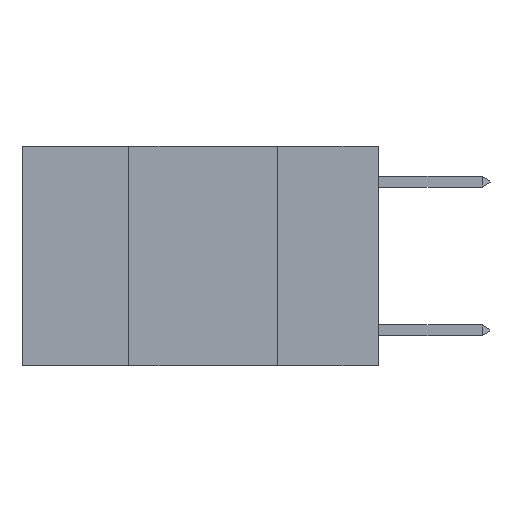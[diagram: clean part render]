
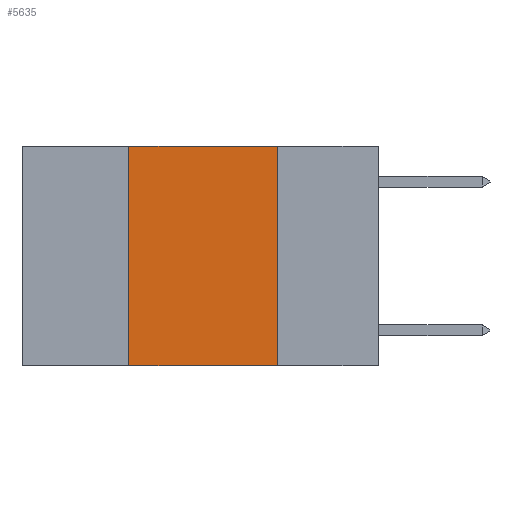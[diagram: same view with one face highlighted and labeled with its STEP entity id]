
A CAD part, left-side view. The second image highlights one B-rep face of the part: STEP entity #5635.
In plain terms, the highlighted planar face has unit normal (-1, 0, 0).
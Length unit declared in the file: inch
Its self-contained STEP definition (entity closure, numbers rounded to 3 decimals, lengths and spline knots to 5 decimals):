
#769 = ORIENTED_EDGE ( 'NONE', *, *, #11869, .F. ) ;
#1101 = LINE ( 'NONE', #7359, #4163 ) ;
#1583 = CARTESIAN_POINT ( 'NONE',  ( 0., 0.6, 0. ) ) ;
#2007 = EDGE_CURVE ( 'NONE', #3129, #12788, #8101, .T. ) ;
#2732 = PLANE ( 'NONE',  #12968 ) ;
#3129 = VERTEX_POINT ( 'NONE', #4435 ) ;
#3573 = VECTOR ( 'NONE', #8600, 39.37008 ) ;
#3729 = EDGE_CURVE ( 'NONE', #4868, #3129, #7641, .T. ) ;
#3752 = ORIENTED_EDGE ( 'NONE', *, *, #3729, .F. ) ;
#4138 = DIRECTION ( 'NONE',  ( 0., -1., 0. ) ) ;
#4163 = VECTOR ( 'NONE', #4138, 39.37008 ) ;
#4435 = CARTESIAN_POINT ( 'NONE',  ( 0., 0.17, 0. ) ) ;
#4826 = DIRECTION ( 'NONE',  ( 0., -1., 0. ) ) ;
#4868 = VERTEX_POINT ( 'NONE', #6043 ) ;
#5635 = ADVANCED_FACE ( 'NONE', ( #6835 ), #2732, .F. ) ;
#5807 = VECTOR ( 'NONE', #4826, 39.37008 ) ;
#5956 = CARTESIAN_POINT ( 'NONE',  ( 0., 0.6, 0. ) ) ;
#6043 = CARTESIAN_POINT ( 'NONE',  ( 0., 0.42, 0. ) ) ;
#6765 = DIRECTION ( 'NONE',  ( 0., 0., -1. ) ) ;
#6835 = FACE_OUTER_BOUND ( 'NONE', #8458, .T. ) ;
#7313 = ORIENTED_EDGE ( 'NONE', *, *, #2007, .F. ) ;
#7359 = CARTESIAN_POINT ( 'NONE',  ( 0., 0.6, -0.37 ) ) ;
#7641 = LINE ( 'NONE', #1583, #5807 ) ;
#8037 = DIRECTION ( 'NONE',  ( 1., 0., 0. ) ) ;
#8101 = LINE ( 'NONE', #11221, #8773 ) ;
#8458 = EDGE_LOOP ( 'NONE', ( #7313, #3752, #769, #10487 ) ) ;
#8600 = DIRECTION ( 'NONE',  ( 0., 0., 1. ) ) ;
#8669 = CARTESIAN_POINT ( 'NONE',  ( 0., 0.42, 0. ) ) ;
#8773 = VECTOR ( 'NONE', #8849, 39.37008 ) ;
#8849 = DIRECTION ( 'NONE',  ( 0., 0., -1. ) ) ;
#9372 = VERTEX_POINT ( 'NONE', #13247 ) ;
#9624 = EDGE_CURVE ( 'NONE', #9372, #12788, #1101, .T. ) ;
#10487 = ORIENTED_EDGE ( 'NONE', *, *, #9624, .T. ) ;
#10651 = LINE ( 'NONE', #8669, #3573 ) ;
#11135 = CARTESIAN_POINT ( 'NONE',  ( 0., 0.17, -0.37 ) ) ;
#11221 = CARTESIAN_POINT ( 'NONE',  ( 0., 0.17, 0. ) ) ;
#11869 = EDGE_CURVE ( 'NONE', #9372, #4868, #10651, .T. ) ;
#12788 = VERTEX_POINT ( 'NONE', #11135 ) ;
#12968 = AXIS2_PLACEMENT_3D ( 'NONE', #5956, #8037, #6765 ) ;
#13247 = CARTESIAN_POINT ( 'NONE',  ( 0., 0.42, -0.37 ) ) ;
